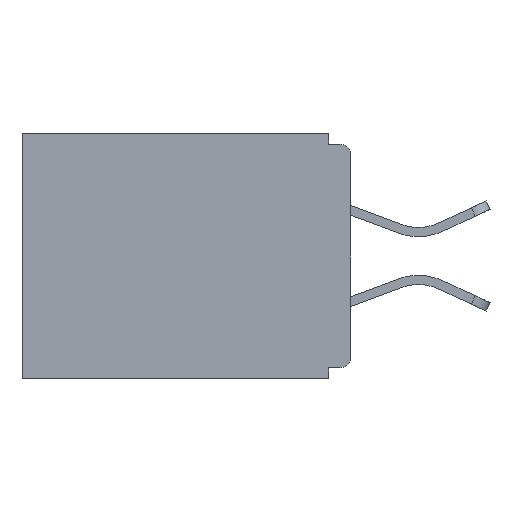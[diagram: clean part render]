
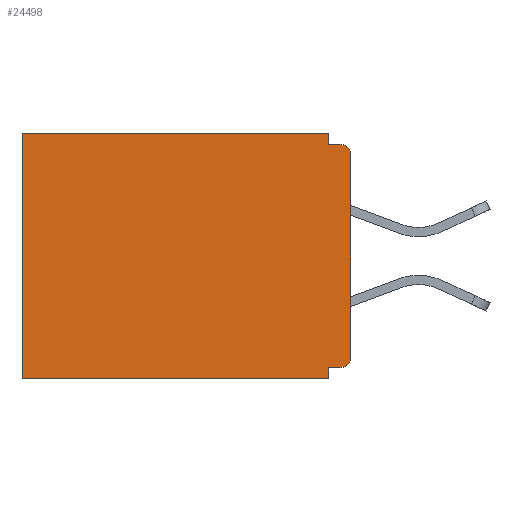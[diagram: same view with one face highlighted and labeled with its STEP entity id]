
A CAD part, left-side view. The second image highlights one B-rep face of the part: STEP entity #24498.
In plain terms, the highlighted planar face has unit normal (-1, 0, 0).
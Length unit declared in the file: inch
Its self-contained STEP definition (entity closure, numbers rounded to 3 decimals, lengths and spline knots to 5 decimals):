
#2 = CARTESIAN_POINT ( 'NONE',  ( 0.298, 0.031, -0.328 ) ) ;
#191 = AXIS2_PLACEMENT_3D ( 'NONE', #19400, #23477, #14464 ) ;
#296 = CARTESIAN_POINT ( 'NONE',  ( 0.298, 0.031, -0.015 ) ) ;
#1082 = CARTESIAN_POINT ( 'NONE',  ( 0.298, 0., 0. ) ) ;
#1182 = ORIENTED_EDGE ( 'NONE', *, *, #6606, .T. ) ;
#1696 = VECTOR ( 'NONE', #15618, 39.37008 ) ;
#1774 = VECTOR ( 'NONE', #14210, 39.37008 ) ;
#1907 = LINE ( 'NONE', #14021, #12035 ) ;
#2407 = CARTESIAN_POINT ( 'NONE',  ( 0.298, 0., -0.343 ) ) ;
#2477 = ORIENTED_EDGE ( 'NONE', *, *, #12295, .T. ) ;
#3003 = EDGE_CURVE ( 'NONE', #12388, #22917, #8405, .T. ) ;
#3307 = CARTESIAN_POINT ( 'NONE',  ( 0.298, 0.031, -0.343 ) ) ;
#3330 = ORIENTED_EDGE ( 'NONE', *, *, #6429, .T. ) ;
#3583 = CARTESIAN_POINT ( 'NONE',  ( 0.298, 0.031, 0. ) ) ;
#3784 = EDGE_CURVE ( 'NONE', #4241, #17268, #12424, .T. ) ;
#4241 = VERTEX_POINT ( 'NONE', #9385 ) ;
#4321 = CARTESIAN_POINT ( 'NONE',  ( 0.298, 0.015, -0.313 ) ) ;
#4722 = EDGE_CURVE ( 'NONE', #10984, #17268, #14598, .T. ) ;
#4746 = VECTOR ( 'NONE', #25908, 39.37008 ) ;
#5977 = CARTESIAN_POINT ( 'NONE',  ( 0.298, 0.46, -0.343 ) ) ;
#6022 = ORIENTED_EDGE ( 'NONE', *, *, #3784, .F. ) ;
#6224 = DIRECTION ( 'NONE',  ( -1., 0., 0. ) ) ;
#6429 = EDGE_CURVE ( 'NONE', #20760, #22917, #18952, .T. ) ;
#6606 = EDGE_CURVE ( 'NONE', #10996, #10984, #22139, .T. ) ;
#6670 = VECTOR ( 'NONE', #11114, 39.37008 ) ;
#7240 = ORIENTED_EDGE ( 'NONE', *, *, #11666, .F. ) ;
#7291 = ORIENTED_EDGE ( 'NONE', *, *, #9802, .F. ) ;
#7423 = VECTOR ( 'NONE', #10076, 39.37008 ) ;
#7929 = EDGE_LOOP ( 'NONE', ( #3330, #14893, #7291, #1182, #12123, #6022, #21496, #7240, #2477, #9708 ) ) ;
#8146 = CIRCLE ( 'NONE', #17812, 0.015 ) ;
#8405 = LINE ( 'NONE', #20323, #7423 ) ;
#9385 = CARTESIAN_POINT ( 'NONE',  ( 0.298, 0.031, -0.343 ) ) ;
#9403 = PLANE ( 'NONE',  #191 ) ;
#9708 = ORIENTED_EDGE ( 'NONE', *, *, #17350, .F. ) ;
#9785 = DIRECTION ( 'NONE',  ( 0., 0., -1. ) ) ;
#9802 = EDGE_CURVE ( 'NONE', #10996, #12388, #11835, .T. ) ;
#10076 = DIRECTION ( 'NONE',  ( 0., -1., 0. ) ) ;
#10321 = FACE_OUTER_BOUND ( 'NONE', #7929, .T. ) ;
#10984 = VERTEX_POINT ( 'NONE', #19983 ) ;
#10996 = VERTEX_POINT ( 'NONE', #3583 ) ;
#11114 = DIRECTION ( 'NONE',  ( 0., 0., -1. ) ) ;
#11666 = EDGE_CURVE ( 'NONE', #19350, #22389, #1907, .T. ) ;
#11835 = LINE ( 'NONE', #3307, #1696 ) ;
#12035 = VECTOR ( 'NONE', #25786, 39.37008 ) ;
#12123 = ORIENTED_EDGE ( 'NONE', *, *, #4722, .T. ) ;
#12282 = AXIS2_PLACEMENT_3D ( 'NONE', #24199, #15881, #9785 ) ;
#12295 = EDGE_CURVE ( 'NONE', #19350, #22881, #8146, .T. ) ;
#12388 = VERTEX_POINT ( 'NONE', #296 ) ;
#12424 = LINE ( 'NONE', #2407, #20017 ) ;
#12487 = DIRECTION ( 'NONE',  ( 0., 0., -1. ) ) ;
#14021 = CARTESIAN_POINT ( 'NONE',  ( 0.298, 0., -0.328 ) ) ;
#14210 = DIRECTION ( 'NONE',  ( 0., 0., -1. ) ) ;
#14279 = CARTESIAN_POINT ( 'NONE',  ( 0.298, 0., -0.313 ) ) ;
#14464 = DIRECTION ( 'NONE',  ( 0., 0., -1. ) ) ;
#14466 = DIRECTION ( 'NONE',  ( 0., 1., 0. ) ) ;
#14598 = LINE ( 'NONE', #23592, #6670 ) ;
#14893 = ORIENTED_EDGE ( 'NONE', *, *, #3003, .F. ) ;
#15155 = EDGE_CURVE ( 'NONE', #22389, #4241, #22500, .T. ) ;
#15618 = DIRECTION ( 'NONE',  ( 0., 0., -1. ) ) ;
#15881 = DIRECTION ( 'NONE',  ( -1., 0., 0. ) ) ;
#16878 = CARTESIAN_POINT ( 'NONE',  ( 0.298, 0., -0.03 ) ) ;
#17268 = VERTEX_POINT ( 'NONE', #5977 ) ;
#17350 = EDGE_CURVE ( 'NONE', #20760, #22881, #19203, .T. ) ;
#17812 = AXIS2_PLACEMENT_3D ( 'NONE', #4321, #6224, #12487 ) ;
#18349 = CARTESIAN_POINT ( 'NONE',  ( 0.298, 0., 0. ) ) ;
#18648 = VECTOR ( 'NONE', #19055, 39.37008 ) ;
#18952 = CIRCLE ( 'NONE', #12282, 0.015 ) ;
#19055 = DIRECTION ( 'NONE',  ( 0., 1., 0. ) ) ;
#19203 = LINE ( 'NONE', #18349, #1774 ) ;
#19350 = VERTEX_POINT ( 'NONE', #25080 ) ;
#19400 = CARTESIAN_POINT ( 'NONE',  ( 0.298, 0., 0. ) ) ;
#19983 = CARTESIAN_POINT ( 'NONE',  ( 0.298, 0.46, 0. ) ) ;
#20017 = VECTOR ( 'NONE', #14466, 39.37008 ) ;
#20323 = CARTESIAN_POINT ( 'NONE',  ( 0.298, 0., -0.015 ) ) ;
#20760 = VERTEX_POINT ( 'NONE', #16878 ) ;
#20810 = CARTESIAN_POINT ( 'NONE',  ( 0.298, 0.015, -0.015 ) ) ;
#21496 = ORIENTED_EDGE ( 'NONE', *, *, #15155, .F. ) ;
#22139 = LINE ( 'NONE', #1082, #18648 ) ;
#22389 = VERTEX_POINT ( 'NONE', #2 ) ;
#22500 = LINE ( 'NONE', #26075, #4746 ) ;
#22881 = VERTEX_POINT ( 'NONE', #14279 ) ;
#22917 = VERTEX_POINT ( 'NONE', #20810 ) ;
#23477 = DIRECTION ( 'NONE',  ( 1., 0., 0. ) ) ;
#23592 = CARTESIAN_POINT ( 'NONE',  ( 0.298, 0.46, 0. ) ) ;
#24199 = CARTESIAN_POINT ( 'NONE',  ( 0.298, 0.015, -0.03 ) ) ;
#24498 = ADVANCED_FACE ( 'NONE', ( #10321 ), #9403, .F. ) ;
#25080 = CARTESIAN_POINT ( 'NONE',  ( 0.298, 0.015, -0.328 ) ) ;
#25786 = DIRECTION ( 'NONE',  ( 0., 1., 0. ) ) ;
#25908 = DIRECTION ( 'NONE',  ( 0., 0., -1. ) ) ;
#26075 = CARTESIAN_POINT ( 'NONE',  ( 0.298, 0.031, -0.343 ) ) ;
